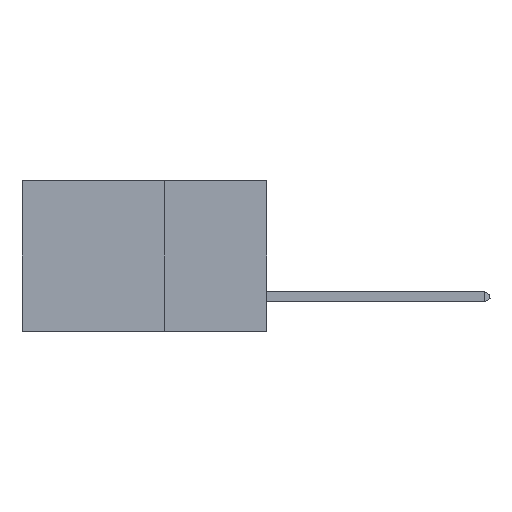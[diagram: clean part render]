
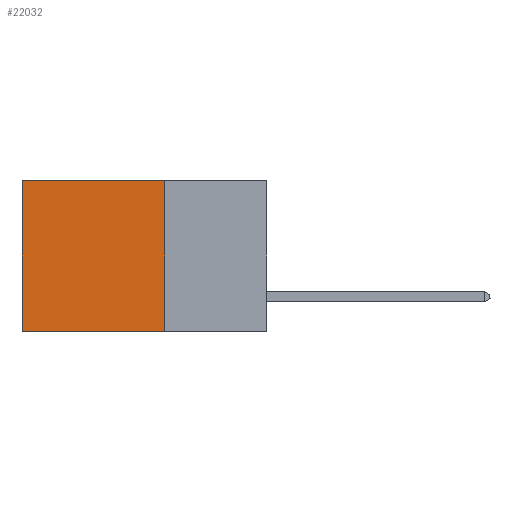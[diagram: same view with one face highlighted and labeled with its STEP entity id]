
A CAD part, left-side view. The second image highlights one B-rep face of the part: STEP entity #22032.
In plain terms, the highlighted planar face has unit normal (-1, 0, 0).
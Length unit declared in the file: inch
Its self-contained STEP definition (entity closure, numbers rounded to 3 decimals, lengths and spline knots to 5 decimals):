
#334 = EDGE_CURVE ( 'NONE', #32163, #17035, #10224, .T. ) ;
#405 = CARTESIAN_POINT ( 'NONE',  ( 0.2875, 0.25, -0.37 ) ) ;
#707 = CARTESIAN_POINT ( 'NONE',  ( 0.2875, 0.25, 0. ) ) ;
#1873 = DIRECTION ( 'NONE',  ( 0., 1., 0. ) ) ;
#2135 = DIRECTION ( 'NONE',  ( 0., 0., -1. ) ) ;
#5763 = DIRECTION ( 'NONE',  ( 0., 1., 0. ) ) ;
#7099 = CARTESIAN_POINT ( 'NONE',  ( 0.2875, 0.25, -0.37 ) ) ;
#8086 = FACE_OUTER_BOUND ( 'NONE', #10830, .T. ) ;
#9429 = VERTEX_POINT ( 'NONE', #19913 ) ;
#10224 = LINE ( 'NONE', #7099, #15844 ) ;
#10830 = EDGE_LOOP ( 'NONE', ( #16832, #26329, #23361, #27316 ) ) ;
#10900 = LINE ( 'NONE', #28176, #12514 ) ;
#11022 = DIRECTION ( 'NONE',  ( 0., 0., -1. ) ) ;
#12514 = VECTOR ( 'NONE', #5763, 39.37008 ) ;
#13093 = VECTOR ( 'NONE', #21007, 39.37008 ) ;
#13782 = AXIS2_PLACEMENT_3D ( 'NONE', #707, #21414, #11022 ) ;
#15844 = VECTOR ( 'NONE', #1873, 39.37008 ) ;
#16160 = CARTESIAN_POINT ( 'NONE',  ( 0.2875, 0.6, -0.37 ) ) ;
#16832 = ORIENTED_EDGE ( 'NONE', *, *, #33229, .T. ) ;
#17035 = VERTEX_POINT ( 'NONE', #16160 ) ;
#17490 = CARTESIAN_POINT ( 'NONE',  ( 0.2875, 0.25, 0. ) ) ;
#18275 = LINE ( 'NONE', #17490, #22335 ) ;
#18751 = LINE ( 'NONE', #20663, #13093 ) ;
#19208 = VERTEX_POINT ( 'NONE', #25816 ) ;
#19523 = EDGE_CURVE ( 'NONE', #9429, #19208, #10900, .T. ) ;
#19913 = CARTESIAN_POINT ( 'NONE',  ( 0.2875, 0.25, 0. ) ) ;
#20663 = CARTESIAN_POINT ( 'NONE',  ( 0.2875, 0.6, 0. ) ) ;
#21007 = DIRECTION ( 'NONE',  ( 0., 0., -1. ) ) ;
#21414 = DIRECTION ( 'NONE',  ( 1., 0., 0. ) ) ;
#22032 = ADVANCED_FACE ( 'NONE', ( #8086 ), #26412, .F. ) ;
#22335 = VECTOR ( 'NONE', #2135, 39.37008 ) ;
#23361 = ORIENTED_EDGE ( 'NONE', *, *, #29559, .F. ) ;
#25816 = CARTESIAN_POINT ( 'NONE',  ( 0.2875, 0.6, 0. ) ) ;
#26329 = ORIENTED_EDGE ( 'NONE', *, *, #334, .F. ) ;
#26412 = PLANE ( 'NONE',  #13782 ) ;
#27316 = ORIENTED_EDGE ( 'NONE', *, *, #19523, .T. ) ;
#28176 = CARTESIAN_POINT ( 'NONE',  ( 0.2875, 0.25, 0. ) ) ;
#29559 = EDGE_CURVE ( 'NONE', #9429, #32163, #18275, .T. ) ;
#32163 = VERTEX_POINT ( 'NONE', #405 ) ;
#33229 = EDGE_CURVE ( 'NONE', #19208, #17035, #18751, .T. ) ;
